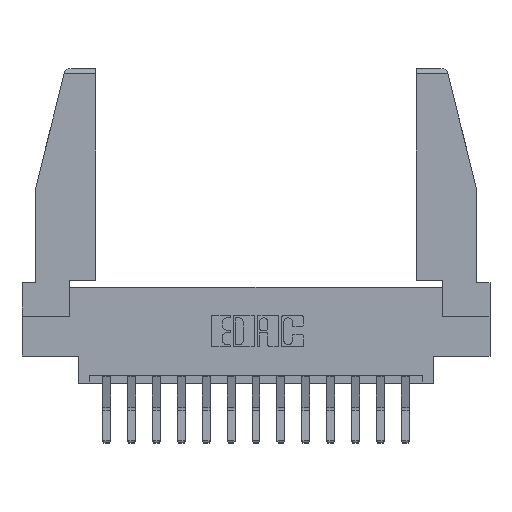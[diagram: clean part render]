
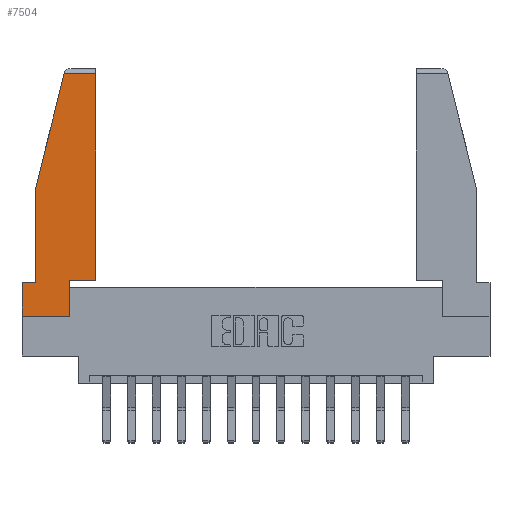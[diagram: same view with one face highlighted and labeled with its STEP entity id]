
A CAD part, top view. The second image highlights one B-rep face of the part: STEP entity #7504.
In plain terms, the highlighted planar face has unit normal (0, 0, 1).
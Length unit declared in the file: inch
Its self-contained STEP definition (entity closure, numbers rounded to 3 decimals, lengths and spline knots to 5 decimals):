
#12 = CARTESIAN_POINT ( 'NONE',  ( 0.461, 0.223, 0. ) ) ;
#198 = ORIENTED_EDGE ( 'NONE', *, *, #6139, .T. ) ;
#353 = DIRECTION ( 'NONE',  ( 1., 0., 0. ) ) ;
#374 = EDGE_CURVE ( 'NONE', #16364, #3002, #2295, .T. ) ;
#1144 = CARTESIAN_POINT ( 'NONE',  ( 0.297, 0., 0. ) ) ;
#1337 = ORIENTED_EDGE ( 'NONE', *, *, #374, .T. ) ;
#1554 = EDGE_CURVE ( 'NONE', #11174, #16364, #7690, .T. ) ;
#1850 = CARTESIAN_POINT ( 'NONE',  ( 0.297, 0.223, 0. ) ) ;
#1929 = ORIENTED_EDGE ( 'NONE', *, *, #11388, .T. ) ;
#2154 = DIRECTION ( 'NONE',  ( 0., -1., 0. ) ) ;
#2295 = LINE ( 'NONE', #3104, #10739 ) ;
#3002 = VERTEX_POINT ( 'NONE', #14269 ) ;
#3052 = VECTOR ( 'NONE', #353, 39.37008 ) ;
#3104 = CARTESIAN_POINT ( 'NONE',  ( 0., 1.52, 0. ) ) ;
#3109 = ORIENTED_EDGE ( 'NONE', *, *, #16067, .T. ) ;
#3361 = VERTEX_POINT ( 'NONE', #3693 ) ;
#3438 = FACE_OUTER_BOUND ( 'NONE', #15394, .T. ) ;
#3693 = CARTESIAN_POINT ( 'NONE',  ( 0.086, 0.8, 0. ) ) ;
#3764 = DIRECTION ( 'NONE',  ( 0., 1., 0. ) ) ;
#3787 = CARTESIAN_POINT ( 'NONE',  ( 0.461, 0.223, 0. ) ) ;
#4097 = CARTESIAN_POINT ( 'NONE',  ( 0., 0.21, 0. ) ) ;
#5451 = LINE ( 'NONE', #6160, #7668 ) ;
#5641 = CARTESIAN_POINT ( 'NONE',  ( 0., 0., 0. ) ) ;
#5999 = CARTESIAN_POINT ( 'NONE',  ( 0., 0., 0. ) ) ;
#6139 = EDGE_CURVE ( 'NONE', #9146, #15912, #13899, .T. ) ;
#6160 = CARTESIAN_POINT ( 'NONE',  ( 0.086, 0.8, 0. ) ) ;
#6217 = VERTEX_POINT ( 'NONE', #1850 ) ;
#6261 = LINE ( 'NONE', #4097, #14075 ) ;
#6268 = LINE ( 'NONE', #10597, #3052 ) ;
#6662 = VERTEX_POINT ( 'NONE', #15242 ) ;
#6883 = EDGE_CURVE ( 'NONE', #7580, #6662, #6261, .T. ) ;
#7001 = CARTESIAN_POINT ( 'NONE',  ( 0.271, 1.55, 0. ) ) ;
#7202 = ORIENTED_EDGE ( 'NONE', *, *, #6883, .T. ) ;
#7275 = EDGE_CURVE ( 'NONE', #6217, #11174, #6268, .T. ) ;
#7451 = LINE ( 'NONE', #1144, #8655 ) ;
#7484 = VECTOR ( 'NONE', #14384, 39.37008 ) ;
#7504 = ADVANCED_FACE ( 'NONE', ( #3438 ), #9875, .T. ) ;
#7576 = CARTESIAN_POINT ( 'NONE',  ( 0., 0., 0. ) ) ;
#7580 = VERTEX_POINT ( 'NONE', #11096 ) ;
#7586 = EDGE_CURVE ( 'NONE', #3361, #7580, #5451, .T. ) ;
#7668 = VECTOR ( 'NONE', #16414, 39.37008 ) ;
#7690 = LINE ( 'NONE', #3787, #7484 ) ;
#7782 = VECTOR ( 'NONE', #2154, 39.37008 ) ;
#7796 = ORIENTED_EDGE ( 'NONE', *, *, #7586, .T. ) ;
#7962 = DIRECTION ( 'NONE',  ( 1., 0., 0. ) ) ;
#8272 = VECTOR ( 'NONE', #15917, 39.37008 ) ;
#8596 = EDGE_CURVE ( 'NONE', #3002, #3361, #10877, .T. ) ;
#8655 = VECTOR ( 'NONE', #3764, 39.37008 ) ;
#8685 = DIRECTION ( 'NONE',  ( 0., 0., 1. ) ) ;
#9146 = VERTEX_POINT ( 'NONE', #5641 ) ;
#9873 = CARTESIAN_POINT ( 'NONE',  ( 0., 0.21, 0. ) ) ;
#9875 = PLANE ( 'NONE',  #10747 ) ;
#10597 = CARTESIAN_POINT ( 'NONE',  ( 0.297, 0.223, 0. ) ) ;
#10739 = VECTOR ( 'NONE', #14486, 39.37008 ) ;
#10747 = AXIS2_PLACEMENT_3D ( 'NONE', #5999, #8685, #14996 ) ;
#10877 = LINE ( 'NONE', #7001, #8272 ) ;
#11096 = CARTESIAN_POINT ( 'NONE',  ( 0.086, 0.21, 0. ) ) ;
#11174 = VERTEX_POINT ( 'NONE', #12 ) ;
#11388 = EDGE_CURVE ( 'NONE', #15912, #6217, #7451, .T. ) ;
#12276 = CARTESIAN_POINT ( 'NONE',  ( 0.297, 0., 0. ) ) ;
#12315 = VECTOR ( 'NONE', #7962, 39.37008 ) ;
#13200 = ORIENTED_EDGE ( 'NONE', *, *, #7275, .T. ) ;
#13697 = ORIENTED_EDGE ( 'NONE', *, *, #8596, .T. ) ;
#13899 = LINE ( 'NONE', #7576, #12315 ) ;
#14075 = VECTOR ( 'NONE', #15724, 39.37008 ) ;
#14269 = CARTESIAN_POINT ( 'NONE',  ( 0.2636, 1.52, 0. ) ) ;
#14291 = ORIENTED_EDGE ( 'NONE', *, *, #1554, .T. ) ;
#14384 = DIRECTION ( 'NONE',  ( 0., 1., 0. ) ) ;
#14486 = DIRECTION ( 'NONE',  ( -1., 0., 0. ) ) ;
#14996 = DIRECTION ( 'NONE',  ( 1., 0., 0. ) ) ;
#15242 = CARTESIAN_POINT ( 'NONE',  ( 0., 0.21, 0. ) ) ;
#15394 = EDGE_LOOP ( 'NONE', ( #14291, #1337, #13697, #7796, #7202, #3109, #198, #1929, #13200 ) ) ;
#15724 = DIRECTION ( 'NONE',  ( -1., 0., 0. ) ) ;
#15912 = VERTEX_POINT ( 'NONE', #12276 ) ;
#15917 = DIRECTION ( 'NONE',  ( -0.239, -0.971, 0. ) ) ;
#15968 = CARTESIAN_POINT ( 'NONE',  ( 0.461, 1.52, 0. ) ) ;
#16067 = EDGE_CURVE ( 'NONE', #6662, #9146, #16355, .T. ) ;
#16355 = LINE ( 'NONE', #9873, #7782 ) ;
#16364 = VERTEX_POINT ( 'NONE', #15968 ) ;
#16414 = DIRECTION ( 'NONE',  ( 0., -1., 0. ) ) ;
